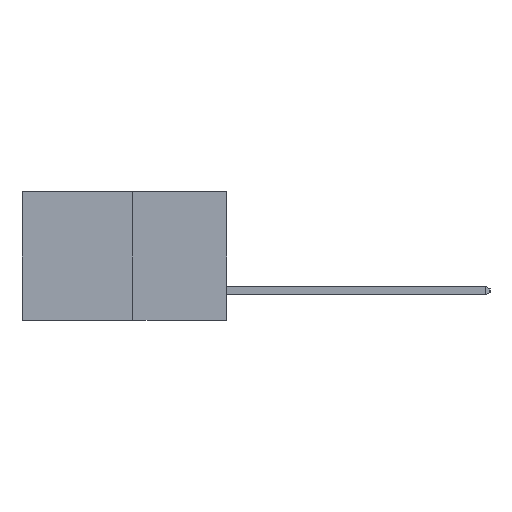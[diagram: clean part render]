
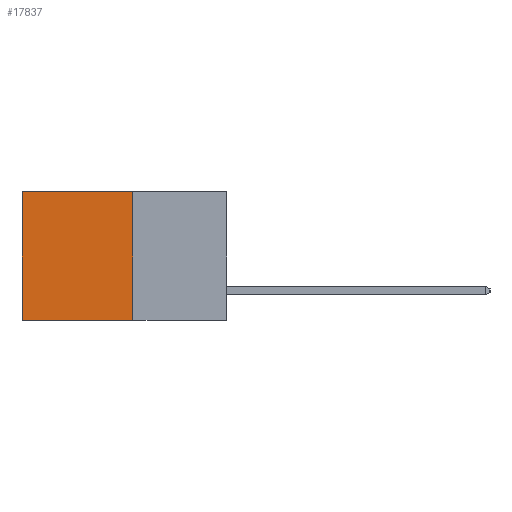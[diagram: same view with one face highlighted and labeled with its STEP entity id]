
A CAD part, left-side view. The second image highlights one B-rep face of the part: STEP entity #17837.
In plain terms, the highlighted planar face has unit normal (-1, 0, 0).
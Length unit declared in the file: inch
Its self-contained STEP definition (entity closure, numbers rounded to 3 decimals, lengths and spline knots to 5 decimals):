
#263 = ORIENTED_EDGE ( 'NONE', *, *, #26426, .T. ) ;
#1252 = PLANE ( 'NONE',  #29760 ) ;
#1262 = ORIENTED_EDGE ( 'NONE', *, *, #20002, .F. ) ;
#1611 = CARTESIAN_POINT ( 'NONE',  ( 0.277, 0.59, -0.37 ) ) ;
#1740 = LINE ( 'NONE', #2296, #26034 ) ;
#2296 = CARTESIAN_POINT ( 'NONE',  ( 0.277, 0.27, 0. ) ) ;
#2958 = VECTOR ( 'NONE', #27927, 39.37008 ) ;
#3590 = VECTOR ( 'NONE', #24178, 39.37008 ) ;
#3655 = DIRECTION ( 'NONE',  ( 1., 0., 0. ) ) ;
#5901 = CARTESIAN_POINT ( 'NONE',  ( 0.277, 0.27, -0.37 ) ) ;
#7064 = VERTEX_POINT ( 'NONE', #5901 ) ;
#9100 = ORIENTED_EDGE ( 'NONE', *, *, #25931, .F. ) ;
#11763 = DIRECTION ( 'NONE',  ( 0., 1., 0. ) ) ;
#13478 = VERTEX_POINT ( 'NONE', #17276 ) ;
#15286 = ORIENTED_EDGE ( 'NONE', *, *, #19678, .T. ) ;
#15545 = LINE ( 'NONE', #25656, #2958 ) ;
#15662 = VERTEX_POINT ( 'NONE', #1611 ) ;
#16453 = CARTESIAN_POINT ( 'NONE',  ( 0.277, 0.59, 0. ) ) ;
#17276 = CARTESIAN_POINT ( 'NONE',  ( 0.277, 0.27, 0. ) ) ;
#17837 = ADVANCED_FACE ( 'NONE', ( #18260 ), #1252, .F. ) ;
#17872 = CARTESIAN_POINT ( 'NONE',  ( 0.277, 0.27, -0.37 ) ) ;
#18260 = FACE_OUTER_BOUND ( 'NONE', #20782, .T. ) ;
#19169 = LINE ( 'NONE', #22676, #24374 ) ;
#19678 = EDGE_CURVE ( 'NONE', #24644, #15662, #15545, .T. ) ;
#20002 = EDGE_CURVE ( 'NONE', #7064, #15662, #19169, .T. ) ;
#20215 = DIRECTION ( 'NONE',  ( 0., 0., -1. ) ) ;
#20782 = EDGE_LOOP ( 'NONE', ( #15286, #1262, #9100, #263 ) ) ;
#21884 = CARTESIAN_POINT ( 'NONE',  ( 0.277, 0.27, -0.37 ) ) ;
#22467 = LINE ( 'NONE', #21884, #3590 ) ;
#22676 = CARTESIAN_POINT ( 'NONE',  ( 0.277, 0.27, -0.37 ) ) ;
#24178 = DIRECTION ( 'NONE',  ( 0., 0., -1. ) ) ;
#24374 = VECTOR ( 'NONE', #29522, 39.37008 ) ;
#24644 = VERTEX_POINT ( 'NONE', #16453 ) ;
#25656 = CARTESIAN_POINT ( 'NONE',  ( 0.277, 0.59, -0.37 ) ) ;
#25931 = EDGE_CURVE ( 'NONE', #13478, #7064, #22467, .T. ) ;
#26034 = VECTOR ( 'NONE', #11763, 39.37008 ) ;
#26426 = EDGE_CURVE ( 'NONE', #13478, #24644, #1740, .T. ) ;
#27927 = DIRECTION ( 'NONE',  ( 0., 0., -1. ) ) ;
#29522 = DIRECTION ( 'NONE',  ( 0., 1., 0. ) ) ;
#29760 = AXIS2_PLACEMENT_3D ( 'NONE', #17872, #3655, #20215 ) ;
